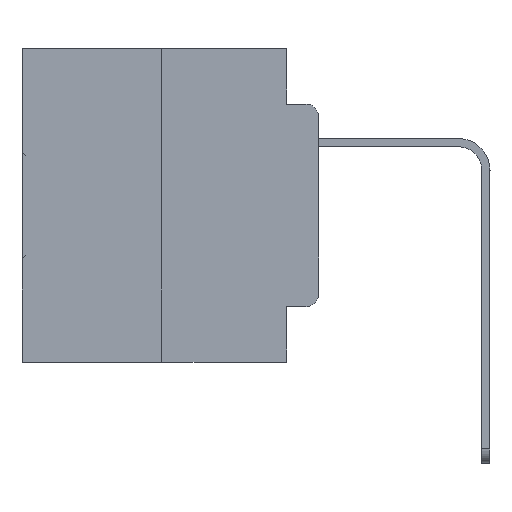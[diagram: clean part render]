
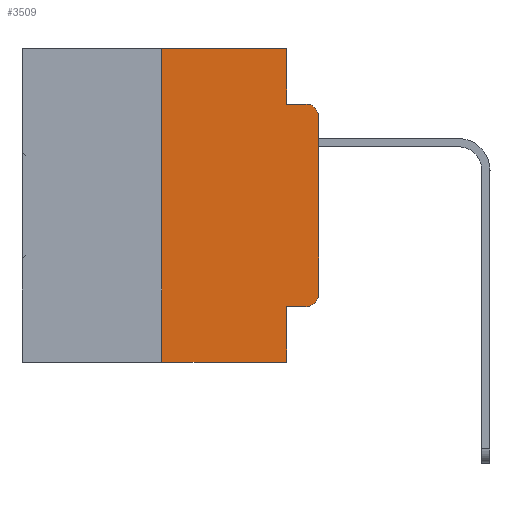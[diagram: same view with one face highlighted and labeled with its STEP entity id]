
A CAD part, left-side view. The second image highlights one B-rep face of the part: STEP entity #3509.
In plain terms, the highlighted planar face has unit normal (-1, 0, 0).
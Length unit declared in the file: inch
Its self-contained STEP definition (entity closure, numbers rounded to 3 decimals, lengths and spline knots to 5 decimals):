
#682 = EDGE_CURVE ( 'NONE', #22523, #1281, #11086, .T. ) ;
#1281 = VERTEX_POINT ( 'NONE', #30440 ) ;
#1448 = EDGE_CURVE ( 'NONE', #23546, #8325, #11396, .T. ) ;
#1703 = CARTESIAN_POINT ( 'NONE',  ( 0., 0.051, 0. ) ) ;
#2731 = DIRECTION ( 'NONE',  ( 0., -1., 0. ) ) ;
#2924 = DIRECTION ( 'NONE',  ( 0., 0., 1. ) ) ;
#3289 = VERTEX_POINT ( 'NONE', #13379 ) ;
#3485 = CARTESIAN_POINT ( 'NONE',  ( 0., 0.051, 0. ) ) ;
#3509 = ADVANCED_FACE ( 'NONE', ( #28791 ), #4990, .F. ) ;
#3988 = EDGE_CURVE ( 'NONE', #13009, #4710, #28535, .T. ) ;
#4710 = VERTEX_POINT ( 'NONE', #8694 ) ;
#4990 = PLANE ( 'NONE',  #8644 ) ;
#5538 = DIRECTION ( 'NONE',  ( 0., 0., -1. ) ) ;
#5544 = ORIENTED_EDGE ( 'NONE', *, *, #23489, .F. ) ;
#5661 = VECTOR ( 'NONE', #28292, 39.37008 ) ;
#5692 = CARTESIAN_POINT ( 'NONE',  ( 0., 0., 0. ) ) ;
#5724 = CARTESIAN_POINT ( 'NONE',  ( 0., 0.25, 0. ) ) ;
#5951 = ORIENTED_EDGE ( 'NONE', *, *, #3988, .T. ) ;
#6305 = DIRECTION ( 'NONE',  ( -1., 0., 0. ) ) ;
#6384 = VERTEX_POINT ( 'NONE', #20613 ) ;
#6929 = VECTOR ( 'NONE', #28044, 39.37008 ) ;
#6953 = LINE ( 'NONE', #1703, #25537 ) ;
#7275 = ORIENTED_EDGE ( 'NONE', *, *, #20027, .F. ) ;
#7443 = DIRECTION ( 'NONE',  ( 0., 0., -1. ) ) ;
#7628 = ORIENTED_EDGE ( 'NONE', *, *, #682, .T. ) ;
#8325 = VERTEX_POINT ( 'NONE', #31382 ) ;
#8644 = AXIS2_PLACEMENT_3D ( 'NONE', #17067, #19617, #26836 ) ;
#8694 = CARTESIAN_POINT ( 'NONE',  ( 0., 0.02, -0.0885 ) ) ;
#9715 = VECTOR ( 'NONE', #14389, 39.37008 ) ;
#10567 = DIRECTION ( 'NONE',  ( 0., 0., -1. ) ) ;
#11086 = LINE ( 'NONE', #25818, #6929 ) ;
#11396 = CIRCLE ( 'NONE', #27236, 0.02 ) ;
#11865 = EDGE_CURVE ( 'NONE', #14908, #23546, #19556, .T. ) ;
#12011 = LINE ( 'NONE', #17020, #9715 ) ;
#12812 = CARTESIAN_POINT ( 'NONE',  ( 0., 0.051, -0.4115 ) ) ;
#13009 = VERTEX_POINT ( 'NONE', #19515 ) ;
#13379 = CARTESIAN_POINT ( 'NONE',  ( 0., 0.051, -0.0885 ) ) ;
#13971 = ORIENTED_EDGE ( 'NONE', *, *, #18179, .F. ) ;
#14389 = DIRECTION ( 'NONE',  ( 0., -1., 0. ) ) ;
#14908 = VERTEX_POINT ( 'NONE', #12812 ) ;
#15665 = VECTOR ( 'NONE', #2924, 39.37008 ) ;
#16121 = DIRECTION ( 'NONE',  ( 0., 0., -1. ) ) ;
#17020 = CARTESIAN_POINT ( 'NONE',  ( 0., 0.473, 0. ) ) ;
#17067 = CARTESIAN_POINT ( 'NONE',  ( 0., 0.473, 0. ) ) ;
#17185 = LINE ( 'NONE', #5692, #15665 ) ;
#18020 = ORIENTED_EDGE ( 'NONE', *, *, #26485, .F. ) ;
#18179 = EDGE_CURVE ( 'NONE', #6384, #23786, #12011, .T. ) ;
#19234 = EDGE_CURVE ( 'NONE', #8325, #13009, #17185, .T. ) ;
#19515 = CARTESIAN_POINT ( 'NONE',  ( 0., 0., -0.1085 ) ) ;
#19556 = LINE ( 'NONE', #19797, #27903 ) ;
#19617 = DIRECTION ( 'NONE',  ( 1., 0., 0. ) ) ;
#19797 = CARTESIAN_POINT ( 'NONE',  ( 0., 0.051, -0.4115 ) ) ;
#19819 = DIRECTION ( 'NONE',  ( -1., 0., 0. ) ) ;
#19868 = CARTESIAN_POINT ( 'NONE',  ( 0., 0.25, -0.5 ) ) ;
#20027 = EDGE_CURVE ( 'NONE', #14908, #1281, #6953, .T. ) ;
#20334 = ORIENTED_EDGE ( 'NONE', *, *, #25359, .F. ) ;
#20613 = CARTESIAN_POINT ( 'NONE',  ( 0., 0.25, 0. ) ) ;
#20918 = EDGE_LOOP ( 'NONE', ( #21541, #5951, #5544, #18020, #13971, #20334, #7628, #7275, #27970, #26817 ) ) ;
#21033 = VECTOR ( 'NONE', #5538, 39.37008 ) ;
#21163 = CARTESIAN_POINT ( 'NONE',  ( 0., 0.051, -0.0885 ) ) ;
#21493 = VECTOR ( 'NONE', #25111, 39.37008 ) ;
#21541 = ORIENTED_EDGE ( 'NONE', *, *, #19234, .T. ) ;
#21915 = CARTESIAN_POINT ( 'NONE',  ( 0., 0.051, 0. ) ) ;
#22266 = CARTESIAN_POINT ( 'NONE',  ( 0., 0.02, -0.3915 ) ) ;
#22410 = CARTESIAN_POINT ( 'NONE',  ( 0., 0.02, -0.1085 ) ) ;
#22523 = VERTEX_POINT ( 'NONE', #19868 ) ;
#23489 = EDGE_CURVE ( 'NONE', #3289, #4710, #28558, .T. ) ;
#23546 = VERTEX_POINT ( 'NONE', #30943 ) ;
#23786 = VERTEX_POINT ( 'NONE', #21915 ) ;
#25111 = DIRECTION ( 'NONE',  ( 0., 0., 1. ) ) ;
#25359 = EDGE_CURVE ( 'NONE', #22523, #6384, #30233, .T. ) ;
#25537 = VECTOR ( 'NONE', #16121, 39.37008 ) ;
#25818 = CARTESIAN_POINT ( 'NONE',  ( 0., 0.473, -0.5 ) ) ;
#26485 = EDGE_CURVE ( 'NONE', #23786, #3289, #26745, .T. ) ;
#26745 = LINE ( 'NONE', #3485, #21033 ) ;
#26817 = ORIENTED_EDGE ( 'NONE', *, *, #1448, .T. ) ;
#26836 = DIRECTION ( 'NONE',  ( 0., 0., -1. ) ) ;
#27236 = AXIS2_PLACEMENT_3D ( 'NONE', #22266, #19819, #7443 ) ;
#27903 = VECTOR ( 'NONE', #2731, 39.37008 ) ;
#27970 = ORIENTED_EDGE ( 'NONE', *, *, #11865, .T. ) ;
#28044 = DIRECTION ( 'NONE',  ( 0., -1., 0. ) ) ;
#28292 = DIRECTION ( 'NONE',  ( 0., -1., 0. ) ) ;
#28535 = CIRCLE ( 'NONE', #28810, 0.02 ) ;
#28558 = LINE ( 'NONE', #21163, #5661 ) ;
#28791 = FACE_OUTER_BOUND ( 'NONE', #20918, .T. ) ;
#28810 = AXIS2_PLACEMENT_3D ( 'NONE', #22410, #6305, #10567 ) ;
#30233 = LINE ( 'NONE', #5724, #21493 ) ;
#30440 = CARTESIAN_POINT ( 'NONE',  ( 0., 0.051, -0.5 ) ) ;
#30943 = CARTESIAN_POINT ( 'NONE',  ( 0., 0.02, -0.4115 ) ) ;
#31382 = CARTESIAN_POINT ( 'NONE',  ( 0., 0., -0.3915 ) ) ;
